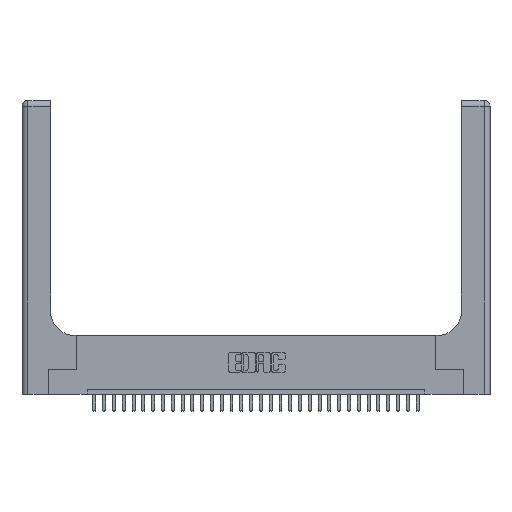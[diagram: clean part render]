
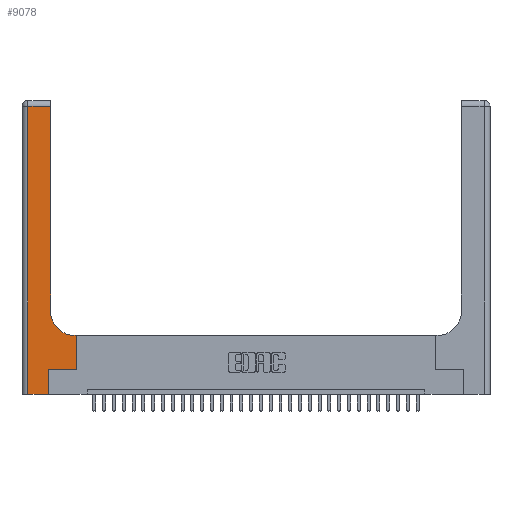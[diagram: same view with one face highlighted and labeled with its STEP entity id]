
A CAD part, top view. The second image highlights one B-rep face of the part: STEP entity #9078.
In plain terms, the highlighted planar face has unit normal (0, 0, 1).
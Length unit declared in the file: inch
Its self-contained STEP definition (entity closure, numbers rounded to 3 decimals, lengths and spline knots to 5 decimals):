
#826 = CARTESIAN_POINT ( 'NONE',  ( 0.2915, 2.94, 0.37 ) ) ;
#840 = PLANE ( 'NONE',  #28861 ) ;
#1554 = EDGE_CURVE ( 'NONE', #5478, #18343, #29999, .T. ) ;
#2157 = CARTESIAN_POINT ( 'NONE',  ( 0.5415, 0.6, 0.37 ) ) ;
#2293 = FACE_OUTER_BOUND ( 'NONE', #25671, .T. ) ;
#2966 = DIRECTION ( 'NONE',  ( 0., 1., 0. ) ) ;
#4430 = CARTESIAN_POINT ( 'NONE',  ( 0.06, 3., 0.37 ) ) ;
#5478 = VERTEX_POINT ( 'NONE', #6540 ) ;
#5747 = CIRCLE ( 'NONE', #18287, 0.25 ) ;
#5904 = CARTESIAN_POINT ( 'NONE',  ( 0.5415, 0.85, 0.37 ) ) ;
#6045 = CARTESIAN_POINT ( 'NONE',  ( 0., 2.94, 0.37 ) ) ;
#6092 = CARTESIAN_POINT ( 'NONE',  ( 0.269, 0., 0.37 ) ) ;
#6488 = EDGE_CURVE ( 'NONE', #6622, #12667, #11186, .T. ) ;
#6540 = CARTESIAN_POINT ( 'NONE',  ( 0.2915, 0.85, 0.37 ) ) ;
#6622 = VERTEX_POINT ( 'NONE', #25894 ) ;
#7259 = CARTESIAN_POINT ( 'NONE',  ( 0.5585, 0.25, 0.37 ) ) ;
#7415 = EDGE_CURVE ( 'NONE', #13015, #5478, #5747, .T. ) ;
#8345 = VERTEX_POINT ( 'NONE', #26141 ) ;
#8584 = EDGE_CURVE ( 'NONE', #11460, #20936, #12341, .T. ) ;
#8810 = VECTOR ( 'NONE', #24227, 39.37008 ) ;
#9078 = ADVANCED_FACE ( 'NONE', ( #2293 ), #840, .F. ) ;
#9702 = DIRECTION ( 'NONE',  ( 0., 1., 0. ) ) ;
#10573 = DIRECTION ( 'NONE',  ( -1., 0., 0. ) ) ;
#10820 = CARTESIAN_POINT ( 'NONE',  ( 0.5585, 0.6, 0.37 ) ) ;
#11186 = LINE ( 'NONE', #14767, #23893 ) ;
#11356 = VECTOR ( 'NONE', #10573, 39.37008 ) ;
#11460 = VERTEX_POINT ( 'NONE', #7259 ) ;
#11866 = DIRECTION ( 'NONE',  ( 1., 0., 0. ) ) ;
#12341 = LINE ( 'NONE', #21761, #26202 ) ;
#12667 = VERTEX_POINT ( 'NONE', #16320 ) ;
#12901 = EDGE_CURVE ( 'NONE', #8345, #6622, #24562, .T. ) ;
#13015 = VERTEX_POINT ( 'NONE', #2157 ) ;
#13164 = VECTOR ( 'NONE', #20802, 39.37008 ) ;
#13590 = ORIENTED_EDGE ( 'NONE', *, *, #8584, .T. ) ;
#14379 = LINE ( 'NONE', #24112, #17043 ) ;
#14444 = LINE ( 'NONE', #6045, #11356 ) ;
#14510 = ORIENTED_EDGE ( 'NONE', *, *, #18730, .T. ) ;
#14767 = CARTESIAN_POINT ( 'NONE',  ( 0., 0., 0.37 ) ) ;
#15489 = VECTOR ( 'NONE', #23228, 39.37008 ) ;
#15822 = DIRECTION ( 'NONE',  ( 1., 0., 0. ) ) ;
#16277 = DIRECTION ( 'NONE',  ( 0., 0., -1. ) ) ;
#16320 = CARTESIAN_POINT ( 'NONE',  ( 0.269, 0., 0.37 ) ) ;
#16973 = CARTESIAN_POINT ( 'NONE',  ( 0.269, 0.25, 0.37 ) ) ;
#17043 = VECTOR ( 'NONE', #11866, 39.37008 ) ;
#17645 = CARTESIAN_POINT ( 'NONE',  ( 0.2915, 3., 0.37 ) ) ;
#18142 = CARTESIAN_POINT ( 'NONE',  ( 0.2915, 0.6, 0.37 ) ) ;
#18179 = ORIENTED_EDGE ( 'NONE', *, *, #6488, .T. ) ;
#18287 = AXIS2_PLACEMENT_3D ( 'NONE', #5904, #20874, #15822 ) ;
#18343 = VERTEX_POINT ( 'NONE', #826 ) ;
#18505 = ORIENTED_EDGE ( 'NONE', *, *, #24664, .T. ) ;
#18730 = EDGE_CURVE ( 'NONE', #27986, #11460, #14379, .T. ) ;
#18955 = LINE ( 'NONE', #18142, #13164 ) ;
#19329 = EDGE_CURVE ( 'NONE', #20936, #13015, #18955, .T. ) ;
#20000 = ORIENTED_EDGE ( 'NONE', *, *, #7415, .T. ) ;
#20584 = CARTESIAN_POINT ( 'NONE',  ( 0., 3., 0.37 ) ) ;
#20802 = DIRECTION ( 'NONE',  ( -1., 0., 0. ) ) ;
#20874 = DIRECTION ( 'NONE',  ( 0., 0., -1. ) ) ;
#20936 = VERTEX_POINT ( 'NONE', #10820 ) ;
#21131 = VECTOR ( 'NONE', #2966, 39.37008 ) ;
#21761 = CARTESIAN_POINT ( 'NONE',  ( 0.5585, 0.25, 0.37 ) ) ;
#22049 = LINE ( 'NONE', #6092, #15489 ) ;
#23225 = ORIENTED_EDGE ( 'NONE', *, *, #31843, .T. ) ;
#23228 = DIRECTION ( 'NONE',  ( 0., 1., 0. ) ) ;
#23893 = VECTOR ( 'NONE', #30450, 39.37008 ) ;
#24112 = CARTESIAN_POINT ( 'NONE',  ( 0.269, 0.25, 0.37 ) ) ;
#24227 = DIRECTION ( 'NONE',  ( 0., -1., 0. ) ) ;
#24562 = LINE ( 'NONE', #4430, #8810 ) ;
#24664 = EDGE_CURVE ( 'NONE', #18343, #8345, #14444, .T. ) ;
#25527 = ORIENTED_EDGE ( 'NONE', *, *, #19329, .T. ) ;
#25671 = EDGE_LOOP ( 'NONE', ( #31750, #18505, #28737, #18179, #23225, #14510, #13590, #25527, #20000 ) ) ;
#25894 = CARTESIAN_POINT ( 'NONE',  ( 0.06, 0., 0.37 ) ) ;
#26141 = CARTESIAN_POINT ( 'NONE',  ( 0.06, 2.94, 0.37 ) ) ;
#26202 = VECTOR ( 'NONE', #9702, 39.37008 ) ;
#26407 = DIRECTION ( 'NONE',  ( -1., 0., 0. ) ) ;
#27986 = VERTEX_POINT ( 'NONE', #16973 ) ;
#28737 = ORIENTED_EDGE ( 'NONE', *, *, #12901, .T. ) ;
#28861 = AXIS2_PLACEMENT_3D ( 'NONE', #20584, #16277, #26407 ) ;
#29999 = LINE ( 'NONE', #17645, #21131 ) ;
#30450 = DIRECTION ( 'NONE',  ( 1., 0., 0. ) ) ;
#31750 = ORIENTED_EDGE ( 'NONE', *, *, #1554, .T. ) ;
#31843 = EDGE_CURVE ( 'NONE', #12667, #27986, #22049, .T. ) ;
